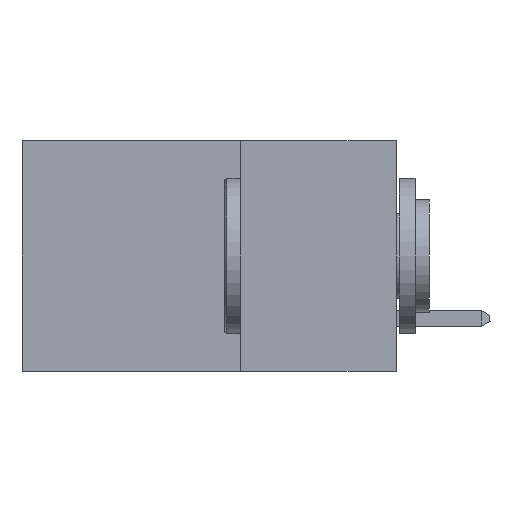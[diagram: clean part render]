
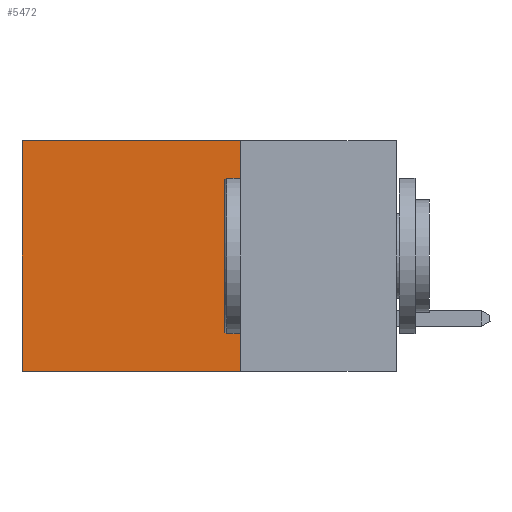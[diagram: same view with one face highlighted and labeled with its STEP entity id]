
A CAD part, left-side view. The second image highlights one B-rep face of the part: STEP entity #5472.
In plain terms, the highlighted planar face has unit normal (-1, 0, 0).
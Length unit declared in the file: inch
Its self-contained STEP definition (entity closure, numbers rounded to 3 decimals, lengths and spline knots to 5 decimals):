
#267 = VERTEX_POINT ( 'NONE', #5024 ) ;
#482 = VECTOR ( 'NONE', #1719, 39.37008 ) ;
#538 = CARTESIAN_POINT ( 'NONE',  ( 0.298, 0.6, 0. ) ) ;
#633 = DIRECTION ( 'NONE',  ( 0., 0., -1. ) ) ;
#666 = CARTESIAN_POINT ( 'NONE',  ( 0.298, 0.25, 0. ) ) ;
#1255 = VERTEX_POINT ( 'NONE', #10884 ) ;
#1260 = VERTEX_POINT ( 'NONE', #8371 ) ;
#1503 = DIRECTION ( 'NONE',  ( 0., 1., 0. ) ) ;
#1719 = DIRECTION ( 'NONE',  ( 0., 1., 0. ) ) ;
#1898 = FACE_OUTER_BOUND ( 'NONE', #9184, .T. ) ;
#2782 = VECTOR ( 'NONE', #3320, 39.37008 ) ;
#3320 = DIRECTION ( 'NONE',  ( 0., 0., -1. ) ) ;
#4149 = ORIENTED_EDGE ( 'NONE', *, *, #11412, .T. ) ;
#4162 = VECTOR ( 'NONE', #633, 39.37008 ) ;
#4280 = CARTESIAN_POINT ( 'NONE',  ( 0.298, 0.6, -0.37 ) ) ;
#4361 = ORIENTED_EDGE ( 'NONE', *, *, #4765, .F. ) ;
#4446 = CARTESIAN_POINT ( 'NONE',  ( 0.298, 0.25, -0.37 ) ) ;
#4680 = DIRECTION ( 'NONE',  ( 1., 0., 0. ) ) ;
#4765 = EDGE_CURVE ( 'NONE', #267, #6216, #7799, .T. ) ;
#5024 = CARTESIAN_POINT ( 'NONE',  ( 0.298, 0.25, -0.37 ) ) ;
#5472 = ADVANCED_FACE ( 'NONE', ( #1898 ), #8426, .F. ) ;
#6216 = VERTEX_POINT ( 'NONE', #4280 ) ;
#6424 = EDGE_CURVE ( 'NONE', #1255, #1260, #8179, .T. ) ;
#6875 = CARTESIAN_POINT ( 'NONE',  ( 0.298, 0.25, 0. ) ) ;
#7799 = LINE ( 'NONE', #4446, #482 ) ;
#7853 = AXIS2_PLACEMENT_3D ( 'NONE', #6875, #4680, #7995 ) ;
#7995 = DIRECTION ( 'NONE',  ( 0., 0., -1. ) ) ;
#8179 = LINE ( 'NONE', #11184, #10236 ) ;
#8371 = CARTESIAN_POINT ( 'NONE',  ( 0.298, 0.6, 0. ) ) ;
#8426 = PLANE ( 'NONE',  #7853 ) ;
#8934 = LINE ( 'NONE', #666, #4162 ) ;
#9184 = EDGE_LOOP ( 'NONE', ( #4149, #4361, #10308, #9640 ) ) ;
#9640 = ORIENTED_EDGE ( 'NONE', *, *, #6424, .T. ) ;
#10236 = VECTOR ( 'NONE', #1503, 39.37008 ) ;
#10281 = LINE ( 'NONE', #538, #2782 ) ;
#10308 = ORIENTED_EDGE ( 'NONE', *, *, #10362, .F. ) ;
#10362 = EDGE_CURVE ( 'NONE', #1255, #267, #8934, .T. ) ;
#10884 = CARTESIAN_POINT ( 'NONE',  ( 0.298, 0.25, 0. ) ) ;
#11184 = CARTESIAN_POINT ( 'NONE',  ( 0.298, 0.25, 0. ) ) ;
#11412 = EDGE_CURVE ( 'NONE', #1260, #6216, #10281, .T. ) ;
